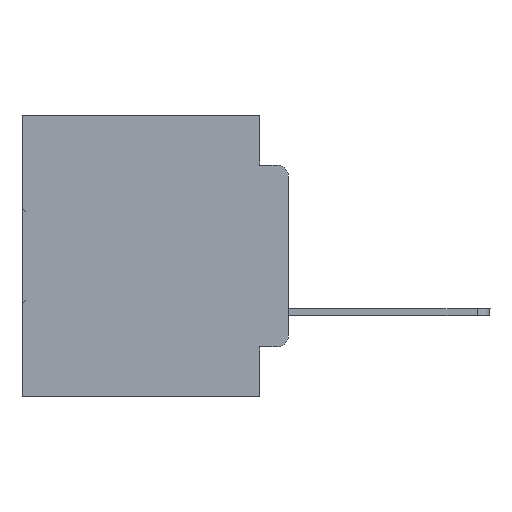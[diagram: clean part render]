
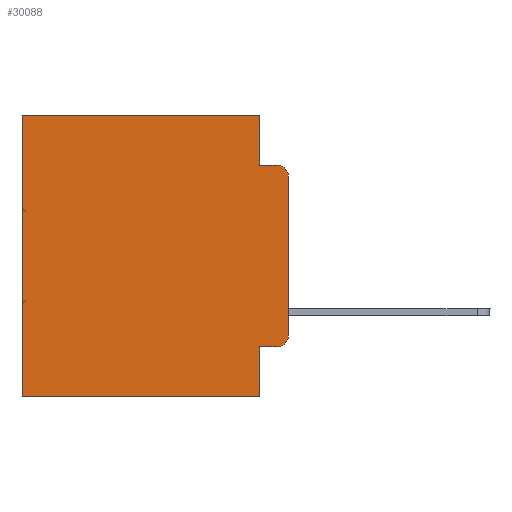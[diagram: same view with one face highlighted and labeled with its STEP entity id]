
A CAD part, left-side view. The second image highlights one B-rep face of the part: STEP entity #30088.
In plain terms, the highlighted planar face has unit normal (-1, 0, 0).
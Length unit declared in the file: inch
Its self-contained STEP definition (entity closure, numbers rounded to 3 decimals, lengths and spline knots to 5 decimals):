
#29 = DIRECTION ( 'NONE',  ( 0., -1., 0. ) ) ;
#139 = VECTOR ( 'NONE', #10125, 39.37008 ) ;
#429 = VERTEX_POINT ( 'NONE', #5886 ) ;
#698 = CIRCLE ( 'NONE', #23264, 0.02 ) ;
#926 = EDGE_CURVE ( 'NONE', #32577, #34215, #698, .T. ) ;
#1239 = VERTEX_POINT ( 'NONE', #30700 ) ;
#2128 = CARTESIAN_POINT ( 'NONE',  ( 0.298, 0.02, -0.4115 ) ) ;
#2145 = LINE ( 'NONE', #10837, #19292 ) ;
#2285 = CARTESIAN_POINT ( 'NONE',  ( 0.298, 0.051, -0.4115 ) ) ;
#2365 = VERTEX_POINT ( 'NONE', #2285 ) ;
#2540 = CARTESIAN_POINT ( 'NONE',  ( 0.298, 0., 0. ) ) ;
#2864 = VECTOR ( 'NONE', #13925, 39.37008 ) ;
#3966 = VECTOR ( 'NONE', #7217, 39.37008 ) ;
#4358 = CARTESIAN_POINT ( 'NONE',  ( 0.298, 0.02, -0.1085 ) ) ;
#4462 = EDGE_CURVE ( 'NONE', #429, #28362, #15284, .T. ) ;
#5520 = CARTESIAN_POINT ( 'NONE',  ( 0.298, 0.051, 0. ) ) ;
#5841 = EDGE_CURVE ( 'NONE', #28362, #34215, #2145, .T. ) ;
#5886 = CARTESIAN_POINT ( 'NONE',  ( 0.298, 0.051, 0. ) ) ;
#6420 = CARTESIAN_POINT ( 'NONE',  ( 0.298, 0.473, 0. ) ) ;
#6519 = ORIENTED_EDGE ( 'NONE', *, *, #16402, .F. ) ;
#7217 = DIRECTION ( 'NONE',  ( 0., -1., 0. ) ) ;
#7413 = LINE ( 'NONE', #6420, #17578 ) ;
#8869 = LINE ( 'NONE', #27780, #30982 ) ;
#9201 = ORIENTED_EDGE ( 'NONE', *, *, #32436, .T. ) ;
#9263 = CARTESIAN_POINT ( 'NONE',  ( 0.298, 0.051, -0.0885 ) ) ;
#10125 = DIRECTION ( 'NONE',  ( 0., 0., -1. ) ) ;
#10837 = CARTESIAN_POINT ( 'NONE',  ( 0.298, 0.051, -0.0885 ) ) ;
#10920 = ORIENTED_EDGE ( 'NONE', *, *, #4462, .F. ) ;
#12035 = CARTESIAN_POINT ( 'NONE',  ( 0.298, 0.051, -0.5 ) ) ;
#12517 = DIRECTION ( 'NONE',  ( -1., 0., 0. ) ) ;
#12535 = VERTEX_POINT ( 'NONE', #12035 ) ;
#13925 = DIRECTION ( 'NONE',  ( 0., 1., 0. ) ) ;
#14461 = CARTESIAN_POINT ( 'NONE',  ( 0.298, 0., -0.5 ) ) ;
#14501 = DIRECTION ( 'NONE',  ( 0., 0., -1. ) ) ;
#14777 = ORIENTED_EDGE ( 'NONE', *, *, #20605, .T. ) ;
#15019 = ORIENTED_EDGE ( 'NONE', *, *, #28755, .F. ) ;
#15154 = PLANE ( 'NONE',  #16953 ) ;
#15284 = LINE ( 'NONE', #25549, #30763 ) ;
#16062 = ORIENTED_EDGE ( 'NONE', *, *, #5841, .F. ) ;
#16402 = EDGE_CURVE ( 'NONE', #2365, #12535, #32407, .T. ) ;
#16953 = AXIS2_PLACEMENT_3D ( 'NONE', #20135, #31104, #31437 ) ;
#17488 = CARTESIAN_POINT ( 'NONE',  ( 0.298, 0.051, -0.4115 ) ) ;
#17578 = VECTOR ( 'NONE', #28981, 39.37008 ) ;
#17925 = EDGE_LOOP ( 'NONE', ( #15019, #19468, #16062, #10920, #9201, #25739, #31668, #6519, #14777, #29530 ) ) ;
#18016 = CIRCLE ( 'NONE', #22543, 0.02 ) ;
#18925 = DIRECTION ( 'NONE',  ( -1., 0., 0. ) ) ;
#19292 = VECTOR ( 'NONE', #29, 39.37008 ) ;
#19468 = ORIENTED_EDGE ( 'NONE', *, *, #926, .T. ) ;
#19768 = LINE ( 'NONE', #14461, #2864 ) ;
#20135 = CARTESIAN_POINT ( 'NONE',  ( 0.298, 0., 0. ) ) ;
#20303 = FACE_OUTER_BOUND ( 'NONE', #17925, .T. ) ;
#20459 = VERTEX_POINT ( 'NONE', #21390 ) ;
#20480 = LINE ( 'NONE', #17488, #3966 ) ;
#20605 = EDGE_CURVE ( 'NONE', #2365, #31119, #20480, .T. ) ;
#21295 = EDGE_CURVE ( 'NONE', #12535, #20459, #19768, .T. ) ;
#21390 = CARTESIAN_POINT ( 'NONE',  ( 0.298, 0.473, -0.5 ) ) ;
#22543 = AXIS2_PLACEMENT_3D ( 'NONE', #26511, #18925, #29714 ) ;
#23264 = AXIS2_PLACEMENT_3D ( 'NONE', #4358, #12517, #23801 ) ;
#23739 = VECTOR ( 'NONE', #34899, 39.37008 ) ;
#23801 = DIRECTION ( 'NONE',  ( 0., 0., -1. ) ) ;
#25549 = CARTESIAN_POINT ( 'NONE',  ( 0.298, 0.051, 0. ) ) ;
#25739 = ORIENTED_EDGE ( 'NONE', *, *, #32689, .T. ) ;
#26511 = CARTESIAN_POINT ( 'NONE',  ( 0.298, 0.02, -0.3915 ) ) ;
#26749 = LINE ( 'NONE', #2540, #23739 ) ;
#27780 = CARTESIAN_POINT ( 'NONE',  ( 0.298, 0., 0. ) ) ;
#28194 = CARTESIAN_POINT ( 'NONE',  ( 0.298, 0., -0.3915 ) ) ;
#28362 = VERTEX_POINT ( 'NONE', #9263 ) ;
#28755 = EDGE_CURVE ( 'NONE', #32577, #32272, #8869, .T. ) ;
#28981 = DIRECTION ( 'NONE',  ( 0., 0., -1. ) ) ;
#29530 = ORIENTED_EDGE ( 'NONE', *, *, #29845, .T. ) ;
#29714 = DIRECTION ( 'NONE',  ( 0., 0., -1. ) ) ;
#29845 = EDGE_CURVE ( 'NONE', #31119, #32272, #18016, .T. ) ;
#30088 = ADVANCED_FACE ( 'NONE', ( #20303 ), #15154, .F. ) ;
#30700 = CARTESIAN_POINT ( 'NONE',  ( 0.298, 0.473, 0. ) ) ;
#30763 = VECTOR ( 'NONE', #33553, 39.37008 ) ;
#30982 = VECTOR ( 'NONE', #14501, 39.37008 ) ;
#31104 = DIRECTION ( 'NONE',  ( 1., 0., 0. ) ) ;
#31119 = VERTEX_POINT ( 'NONE', #2128 ) ;
#31437 = DIRECTION ( 'NONE',  ( 0., 0., -1. ) ) ;
#31668 = ORIENTED_EDGE ( 'NONE', *, *, #21295, .F. ) ;
#32272 = VERTEX_POINT ( 'NONE', #28194 ) ;
#32407 = LINE ( 'NONE', #5520, #139 ) ;
#32436 = EDGE_CURVE ( 'NONE', #429, #1239, #26749, .T. ) ;
#32577 = VERTEX_POINT ( 'NONE', #32596 ) ;
#32596 = CARTESIAN_POINT ( 'NONE',  ( 0.298, 0., -0.1085 ) ) ;
#32689 = EDGE_CURVE ( 'NONE', #1239, #20459, #7413, .T. ) ;
#33553 = DIRECTION ( 'NONE',  ( 0., 0., -1. ) ) ;
#33593 = CARTESIAN_POINT ( 'NONE',  ( 0.298, 0.02, -0.0885 ) ) ;
#34215 = VERTEX_POINT ( 'NONE', #33593 ) ;
#34899 = DIRECTION ( 'NONE',  ( 0., 1., 0. ) ) ;
